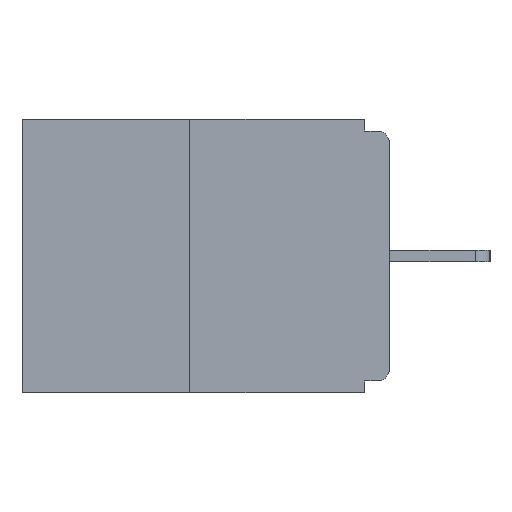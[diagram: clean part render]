
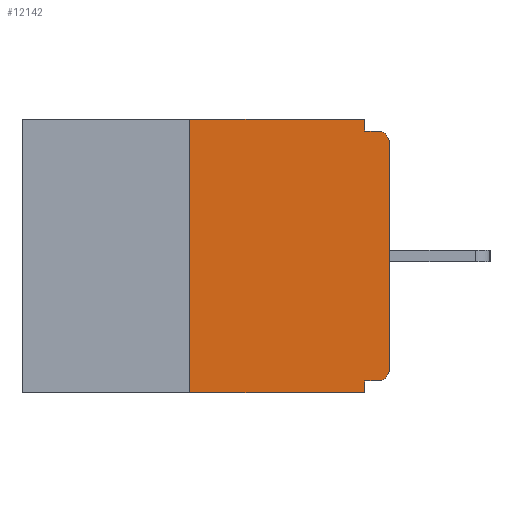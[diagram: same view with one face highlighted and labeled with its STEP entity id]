
A CAD part, left-side view. The second image highlights one B-rep face of the part: STEP entity #12142.
In plain terms, the highlighted planar face has unit normal (-1, 0, 0).
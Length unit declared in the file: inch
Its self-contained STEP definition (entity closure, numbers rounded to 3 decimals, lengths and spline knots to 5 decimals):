
#17 = LINE ( 'NONE', #10372, #10929 ) ;
#226 = DIRECTION ( 'NONE',  ( 0., 0., -1. ) ) ;
#352 = EDGE_CURVE ( 'NONE', #654, #7804, #12034, .T. ) ;
#364 = ORIENTED_EDGE ( 'NONE', *, *, #2317, .F. ) ;
#430 = VERTEX_POINT ( 'NONE', #12252 ) ;
#562 = AXIS2_PLACEMENT_3D ( 'NONE', #5004, #2297, #2352 ) ;
#654 = VERTEX_POINT ( 'NONE', #10956 ) ;
#741 = CARTESIAN_POINT ( 'NONE',  ( 0., 0.25, -0.343 ) ) ;
#860 = VERTEX_POINT ( 'NONE', #741 ) ;
#934 = CARTESIAN_POINT ( 'NONE',  ( 0., 0.46, -0.343 ) ) ;
#1058 = EDGE_CURVE ( 'NONE', #430, #10833, #5303, .T. ) ;
#1063 = CARTESIAN_POINT ( 'NONE',  ( 0., 0.25, 0. ) ) ;
#1431 = VECTOR ( 'NONE', #4837, 39.37008 ) ;
#1493 = DIRECTION ( 'NONE',  ( 0., 0., -1. ) ) ;
#1774 = CARTESIAN_POINT ( 'NONE',  ( 0., 0.031, -0.343 ) ) ;
#1969 = LINE ( 'NONE', #7519, #10549 ) ;
#2103 = DIRECTION ( 'NONE',  ( 1., 0., 0. ) ) ;
#2159 = PLANE ( 'NONE',  #9378 ) ;
#2209 = CARTESIAN_POINT ( 'NONE',  ( 0., 0.031, 0. ) ) ;
#2212 = CARTESIAN_POINT ( 'NONE',  ( 0., 0., -0.313 ) ) ;
#2297 = DIRECTION ( 'NONE',  ( -1., 0., 0. ) ) ;
#2317 = EDGE_CURVE ( 'NONE', #860, #3121, #6812, .T. ) ;
#2352 = DIRECTION ( 'NONE',  ( 0., 0., -1. ) ) ;
#2651 = CARTESIAN_POINT ( 'NONE',  ( 0., 0.031, -0.343 ) ) ;
#2893 = VECTOR ( 'NONE', #9987, 39.37008 ) ;
#2937 = VECTOR ( 'NONE', #5434, 39.37008 ) ;
#3105 = CARTESIAN_POINT ( 'NONE',  ( 0., 0., -0.03 ) ) ;
#3121 = VERTEX_POINT ( 'NONE', #11301 ) ;
#3697 = DIRECTION ( 'NONE',  ( 0., -1., 0. ) ) ;
#3782 = LINE ( 'NONE', #934, #9675 ) ;
#3988 = EDGE_CURVE ( 'NONE', #9108, #10501, #5717, .T. ) ;
#4261 = ORIENTED_EDGE ( 'NONE', *, *, #9646, .T. ) ;
#4264 = EDGE_CURVE ( 'NONE', #10501, #6947, #6203, .T. ) ;
#4288 = CARTESIAN_POINT ( 'NONE',  ( 0., 0., -0.015 ) ) ;
#4332 = DIRECTION ( 'NONE',  ( -1., 0., 0. ) ) ;
#4837 = DIRECTION ( 'NONE',  ( 0., 0., 1. ) ) ;
#5004 = CARTESIAN_POINT ( 'NONE',  ( 0., 0.015, -0.03 ) ) ;
#5033 = EDGE_CURVE ( 'NONE', #7804, #11771, #1969, .T. ) ;
#5127 = ORIENTED_EDGE ( 'NONE', *, *, #352, .T. ) ;
#5303 = LINE ( 'NONE', #2651, #11796 ) ;
#5313 = CIRCLE ( 'NONE', #562, 0.015 ) ;
#5434 = DIRECTION ( 'NONE',  ( 0., 1., 0. ) ) ;
#5486 = EDGE_CURVE ( 'NONE', #3121, #9108, #17, .T. ) ;
#5717 = LINE ( 'NONE', #7624, #11402 ) ;
#6100 = AXIS2_PLACEMENT_3D ( 'NONE', #11716, #4332, #1493 ) ;
#6203 = LINE ( 'NONE', #4288, #2893 ) ;
#6359 = LINE ( 'NONE', #10142, #2937 ) ;
#6478 = ORIENTED_EDGE ( 'NONE', *, *, #4264, .F. ) ;
#6701 = EDGE_CURVE ( 'NONE', #11771, #6947, #5313, .T. ) ;
#6797 = EDGE_CURVE ( 'NONE', #654, #430, #6359, .T. ) ;
#6812 = LINE ( 'NONE', #1063, #1431 ) ;
#6947 = VERTEX_POINT ( 'NONE', #8467 ) ;
#7240 = EDGE_LOOP ( 'NONE', ( #10490, #364, #4261, #11998, #8608, #5127, #10409, #12180, #6478, #9773 ) ) ;
#7519 = CARTESIAN_POINT ( 'NONE',  ( 0., 0., 0. ) ) ;
#7624 = CARTESIAN_POINT ( 'NONE',  ( 0., 0.031, 0. ) ) ;
#7804 = VERTEX_POINT ( 'NONE', #2212 ) ;
#8467 = CARTESIAN_POINT ( 'NONE',  ( 0., 0.015, -0.015 ) ) ;
#8608 = ORIENTED_EDGE ( 'NONE', *, *, #6797, .F. ) ;
#9108 = VERTEX_POINT ( 'NONE', #2209 ) ;
#9259 = DIRECTION ( 'NONE',  ( 0., 0., -1. ) ) ;
#9378 = AXIS2_PLACEMENT_3D ( 'NONE', #9585, #2103, #226 ) ;
#9421 = DIRECTION ( 'NONE',  ( 0., -1., 0. ) ) ;
#9585 = CARTESIAN_POINT ( 'NONE',  ( 0., 0.46, 0. ) ) ;
#9646 = EDGE_CURVE ( 'NONE', #860, #10833, #3782, .T. ) ;
#9675 = VECTOR ( 'NONE', #9421, 39.37008 ) ;
#9773 = ORIENTED_EDGE ( 'NONE', *, *, #3988, .F. ) ;
#9987 = DIRECTION ( 'NONE',  ( 0., -1., 0. ) ) ;
#10011 = CARTESIAN_POINT ( 'NONE',  ( 0., 0.031, -0.015 ) ) ;
#10142 = CARTESIAN_POINT ( 'NONE',  ( 0., 0., -0.328 ) ) ;
#10372 = CARTESIAN_POINT ( 'NONE',  ( 0., 0.46, 0. ) ) ;
#10388 = DIRECTION ( 'NONE',  ( 0., 0., 1. ) ) ;
#10409 = ORIENTED_EDGE ( 'NONE', *, *, #5033, .T. ) ;
#10490 = ORIENTED_EDGE ( 'NONE', *, *, #5486, .F. ) ;
#10501 = VERTEX_POINT ( 'NONE', #10011 ) ;
#10549 = VECTOR ( 'NONE', #10388, 39.37008 ) ;
#10833 = VERTEX_POINT ( 'NONE', #1774 ) ;
#10929 = VECTOR ( 'NONE', #3697, 39.37008 ) ;
#10956 = CARTESIAN_POINT ( 'NONE',  ( 0., 0.015, -0.328 ) ) ;
#11149 = FACE_OUTER_BOUND ( 'NONE', #7240, .T. ) ;
#11301 = CARTESIAN_POINT ( 'NONE',  ( 0., 0.25, 0. ) ) ;
#11304 = DIRECTION ( 'NONE',  ( 0., 0., -1. ) ) ;
#11402 = VECTOR ( 'NONE', #11304, 39.37008 ) ;
#11716 = CARTESIAN_POINT ( 'NONE',  ( 0., 0.015, -0.313 ) ) ;
#11771 = VERTEX_POINT ( 'NONE', #3105 ) ;
#11796 = VECTOR ( 'NONE', #9259, 39.37008 ) ;
#11998 = ORIENTED_EDGE ( 'NONE', *, *, #1058, .F. ) ;
#12034 = CIRCLE ( 'NONE', #6100, 0.015 ) ;
#12142 = ADVANCED_FACE ( 'NONE', ( #11149 ), #2159, .F. ) ;
#12180 = ORIENTED_EDGE ( 'NONE', *, *, #6701, .T. ) ;
#12252 = CARTESIAN_POINT ( 'NONE',  ( 0., 0.031, -0.328 ) ) ;
